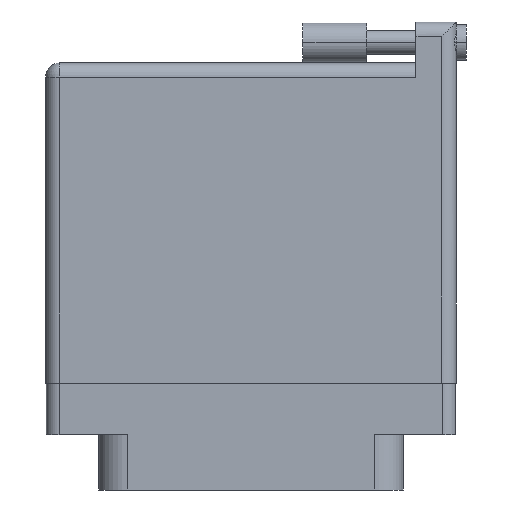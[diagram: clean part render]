
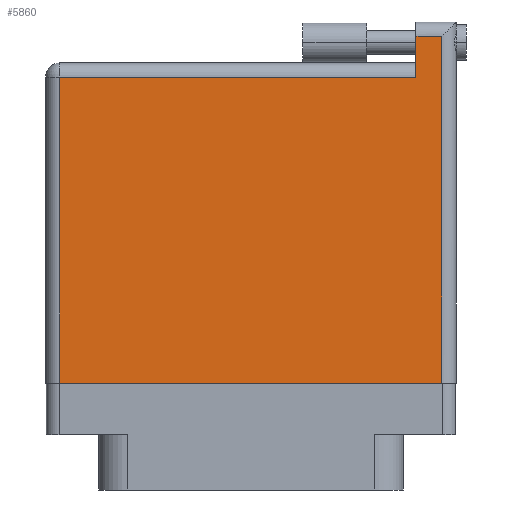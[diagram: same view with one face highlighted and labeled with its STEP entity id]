
A CAD part, front view. The second image highlights one B-rep face of the part: STEP entity #5860.
In plain terms, the highlighted face is planar.
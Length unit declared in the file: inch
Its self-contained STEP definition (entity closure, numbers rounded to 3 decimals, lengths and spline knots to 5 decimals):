
#1999 = CARTESIAN_POINT ( 'NONE',  ( 0.934, 1.596, 0.4495 ) ) ;
#3192 = VERTEX_POINT ( 'NONE', #30607 ) ;
#3284 = EDGE_CURVE ( 'NONE', #16139, #31910, #4414, .T. ) ;
#3544 = DIRECTION ( 'NONE',  ( -1., 0., 0. ) ) ;
#3720 = VERTEX_POINT ( 'NONE', #35756 ) ;
#4414 = LINE ( 'NONE', #33717, #33038 ) ;
#4706 = DIRECTION ( 'NONE',  ( -1., 0., 0. ) ) ;
#5243 = DIRECTION ( 'NONE',  ( -1., 0., 0. ) ) ;
#5761 = EDGE_LOOP ( 'NONE', ( #26639, #8854, #22559, #12481, #22476, #35023 ) ) ;
#5860 = ADVANCED_FACE ( 'NONE', ( #20326 ), #13092, .F. ) ;
#6250 = VERTEX_POINT ( 'NONE', #15512 ) ;
#8854 = ORIENTED_EDGE ( 'NONE', *, *, #15517, .T. ) ;
#9073 = CARTESIAN_POINT ( 'NONE',  ( 0.807, 1.596, 0.4495 ) ) ;
#10277 = LINE ( 'NONE', #34810, #32788 ) ;
#10354 = CARTESIAN_POINT ( 'NONE',  ( -1.004, 1.396, 0.4495 ) ) ;
#11115 = VECTOR ( 'NONE', #25514, 39.37008 ) ;
#11404 = AXIS2_PLACEMENT_3D ( 'NONE', #13952, #24796, #4706 ) ;
#11577 = VERTEX_POINT ( 'NONE', #12345 ) ;
#11890 = CARTESIAN_POINT ( 'NONE',  ( -1.004, -0.1, 0.4495 ) ) ;
#11931 = VECTOR ( 'NONE', #5243, 39.37008 ) ;
#12345 = CARTESIAN_POINT ( 'NONE',  ( -0.934, -0.1, 0.4495 ) ) ;
#12432 = DIRECTION ( 'NONE',  ( 0., 1., 0. ) ) ;
#12481 = ORIENTED_EDGE ( 'NONE', *, *, #27095, .T. ) ;
#13092 = PLANE ( 'NONE',  #11404 ) ;
#13471 = EDGE_CURVE ( 'NONE', #11577, #3720, #32670, .T. ) ;
#13952 = CARTESIAN_POINT ( 'NONE',  ( -1.004, 1.466, 0.4495 ) ) ;
#15512 = CARTESIAN_POINT ( 'NONE',  ( -0.934, 1.396, 0.4495 ) ) ;
#15517 = EDGE_CURVE ( 'NONE', #3720, #16139, #10277, .T. ) ;
#16139 = VERTEX_POINT ( 'NONE', #1999 ) ;
#18797 = LINE ( 'NONE', #25347, #34836 ) ;
#19264 = VECTOR ( 'NONE', #23481, 39.37008 ) ;
#20326 = FACE_OUTER_BOUND ( 'NONE', #5761, .T. ) ;
#22476 = ORIENTED_EDGE ( 'NONE', *, *, #29699, .T. ) ;
#22559 = ORIENTED_EDGE ( 'NONE', *, *, #3284, .T. ) ;
#23481 = DIRECTION ( 'NONE',  ( 1., 0., 0. ) ) ;
#24796 = DIRECTION ( 'NONE',  ( 0., 0., -1. ) ) ;
#24897 = LINE ( 'NONE', #10354, #11931 ) ;
#25245 = DIRECTION ( 'NONE',  ( 0., -1., 0. ) ) ;
#25347 = CARTESIAN_POINT ( 'NONE',  ( -0.934, -0.1, 0.4495 ) ) ;
#25514 = DIRECTION ( 'NONE',  ( 0., -1., 0. ) ) ;
#25795 = LINE ( 'NONE', #33413, #11115 ) ;
#26639 = ORIENTED_EDGE ( 'NONE', *, *, #13471, .T. ) ;
#27095 = EDGE_CURVE ( 'NONE', #31910, #3192, #25795, .T. ) ;
#29699 = EDGE_CURVE ( 'NONE', #3192, #6250, #24897, .T. ) ;
#30607 = CARTESIAN_POINT ( 'NONE',  ( 0.807, 1.396, 0.4495 ) ) ;
#31910 = VERTEX_POINT ( 'NONE', #9073 ) ;
#32670 = LINE ( 'NONE', #11890, #19264 ) ;
#32788 = VECTOR ( 'NONE', #12432, 39.37008 ) ;
#33038 = VECTOR ( 'NONE', #3544, 39.37008 ) ;
#33413 = CARTESIAN_POINT ( 'NONE',  ( 0.807, 1.666, 0.4495 ) ) ;
#33717 = CARTESIAN_POINT ( 'NONE',  ( -1.004, 1.596, 0.4495 ) ) ;
#34810 = CARTESIAN_POINT ( 'NONE',  ( 0.934, 1.666, 0.4495 ) ) ;
#34836 = VECTOR ( 'NONE', #25245, 39.37008 ) ;
#35023 = ORIENTED_EDGE ( 'NONE', *, *, #35140, .T. ) ;
#35140 = EDGE_CURVE ( 'NONE', #6250, #11577, #18797, .T. ) ;
#35756 = CARTESIAN_POINT ( 'NONE',  ( 0.934, -0.1, 0.4495 ) ) ;
